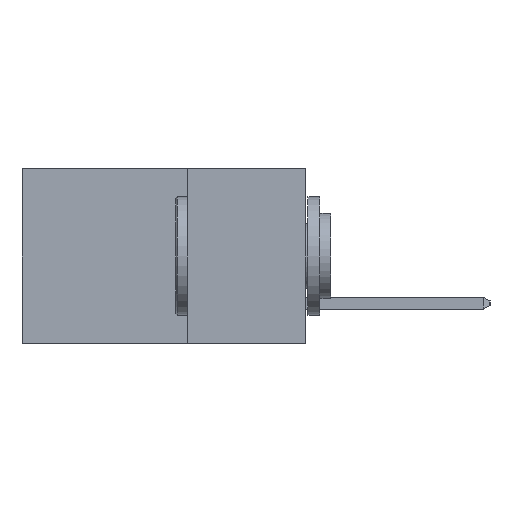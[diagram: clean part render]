
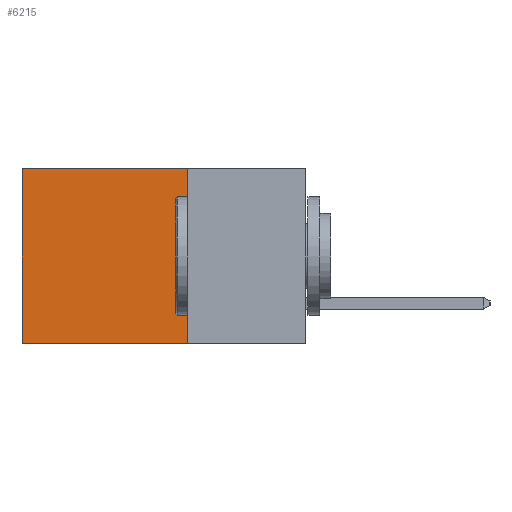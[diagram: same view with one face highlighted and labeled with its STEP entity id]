
A CAD part, left-side view. The second image highlights one B-rep face of the part: STEP entity #6215.
In plain terms, the highlighted planar face has unit normal (-1, 0, 0).
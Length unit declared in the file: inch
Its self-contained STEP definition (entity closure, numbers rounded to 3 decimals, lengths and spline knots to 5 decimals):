
#31 = ORIENTED_EDGE ( 'NONE', *, *, #21706, .T. ) ;
#2178 = ORIENTED_EDGE ( 'NONE', *, *, #3054, .T. ) ;
#2942 = CARTESIAN_POINT ( 'NONE',  ( 0.2615, 0.6, -0.37 ) ) ;
#3054 = EDGE_CURVE ( 'NONE', #6193, #8115, #14649, .T. ) ;
#3637 = CARTESIAN_POINT ( 'NONE',  ( 0.2615, 0.6, -0.37 ) ) ;
#3696 = EDGE_CURVE ( 'NONE', #11373, #14052, #4488, .T. ) ;
#3758 = AXIS2_PLACEMENT_3D ( 'NONE', #6738, #6720, #6694 ) ;
#4488 = LINE ( 'NONE', #15153, #21964 ) ;
#4550 = CARTESIAN_POINT ( 'NONE',  ( 0.2615, 0.6, 0. ) ) ;
#5305 = CARTESIAN_POINT ( 'NONE',  ( 0.2615, 0.25, -0.37 ) ) ;
#5326 = DIRECTION ( 'NONE',  ( 0., 1., 0. ) ) ;
#5718 = VECTOR ( 'NONE', #16798, 39.37008 ) ;
#5841 = CARTESIAN_POINT ( 'NONE',  ( 0.2615, 0.25, 0. ) ) ;
#6193 = VERTEX_POINT ( 'NONE', #8336 ) ;
#6215 = ADVANCED_FACE ( 'NONE', ( #18067 ), #7022, .F. ) ;
#6583 = VECTOR ( 'NONE', #16002, 39.37008 ) ;
#6694 = DIRECTION ( 'NONE',  ( 0., 0., -1. ) ) ;
#6720 = DIRECTION ( 'NONE',  ( 1., 0., 0. ) ) ;
#6738 = CARTESIAN_POINT ( 'NONE',  ( 0.2615, 0.25, -0.37 ) ) ;
#7022 = PLANE ( 'NONE',  #3758 ) ;
#8115 = VERTEX_POINT ( 'NONE', #4550 ) ;
#8336 = CARTESIAN_POINT ( 'NONE',  ( 0.2615, 0.25, 0. ) ) ;
#8466 = ORIENTED_EDGE ( 'NONE', *, *, #3696, .F. ) ;
#8998 = VECTOR ( 'NONE', #5326, 39.37008 ) ;
#11280 = LINE ( 'NONE', #12683, #6583 ) ;
#11373 = VERTEX_POINT ( 'NONE', #5305 ) ;
#12683 = CARTESIAN_POINT ( 'NONE',  ( 0.2615, 0.25, -0.37 ) ) ;
#14052 = VERTEX_POINT ( 'NONE', #3637 ) ;
#14129 = EDGE_CURVE ( 'NONE', #6193, #11373, #11280, .T. ) ;
#14649 = LINE ( 'NONE', #5841, #8998 ) ;
#14909 = DIRECTION ( 'NONE',  ( 0., 1., 0. ) ) ;
#15153 = CARTESIAN_POINT ( 'NONE',  ( 0.2615, 0.25, -0.37 ) ) ;
#16002 = DIRECTION ( 'NONE',  ( 0., 0., -1. ) ) ;
#16798 = DIRECTION ( 'NONE',  ( 0., 0., -1. ) ) ;
#17466 = ORIENTED_EDGE ( 'NONE', *, *, #14129, .F. ) ;
#17879 = EDGE_LOOP ( 'NONE', ( #31, #8466, #17466, #2178 ) ) ;
#18067 = FACE_OUTER_BOUND ( 'NONE', #17879, .T. ) ;
#19316 = LINE ( 'NONE', #2942, #5718 ) ;
#21706 = EDGE_CURVE ( 'NONE', #8115, #14052, #19316, .T. ) ;
#21964 = VECTOR ( 'NONE', #14909, 39.37008 ) ;
